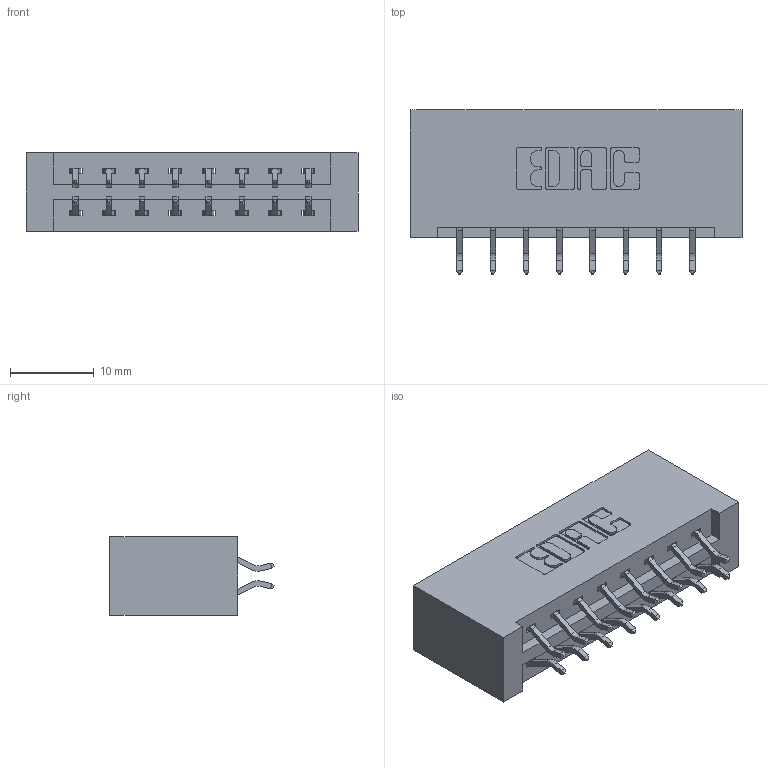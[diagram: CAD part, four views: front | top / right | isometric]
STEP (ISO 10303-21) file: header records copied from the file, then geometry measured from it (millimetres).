
FILE_DESCRIPTION (( 'STEP AP203' ), '1' );
FILE_NAME ('337-016-556-201.STEP', '2018-08-04T20:17:44', ( '' ), ( '' ), 'SwSTEP 2.0', 'SolidWorks 2016', '' );
FILE_SCHEMA (( 'CONFIG_CONTROL_DESIGN' ));
Length unit declared in the file: inch
Products named in the file (3): 337 Part_No Mounting Lugs; 345-292-001_556 Tail; 337-016-556-201
Assembly tree (17 placements, depth 2):
  337-016-556-201
    337 Part_No Mounting Lugs
    345-292-001_556 Tail  x16
Bounding box: 39.57 x 19.57 x 9.4 mm (x, y, z)
Volume: 4478.1 mm3; surface area: 4771.4 mm2
Topology: 17 solids, 17 shells, 1066 faces, 3151 edges, 2078 vertices
Faces by surface type: plane 738, cylinder 328
Entity records: 10543 total; most frequent: CARTESIAN_POINT 1818, ORIENTED_EDGE 1742, DIRECTION 1591, EDGE_CURVE 871, LINE 743, VECTOR 743, VERTEX_POINT 578, AXIS2_PLACEMENT_3D 424
